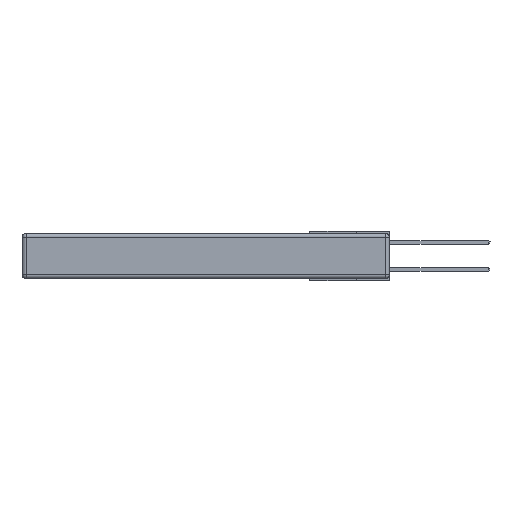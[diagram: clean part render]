
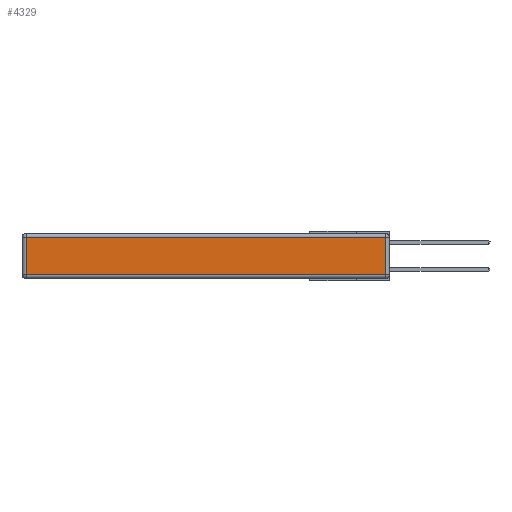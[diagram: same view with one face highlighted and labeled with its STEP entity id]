
A CAD part, left-side view. The second image highlights one B-rep face of the part: STEP entity #4329.
In plain terms, the highlighted planar face has unit normal (-1, 0, 0).
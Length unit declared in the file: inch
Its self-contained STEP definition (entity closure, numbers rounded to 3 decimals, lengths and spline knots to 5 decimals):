
#688 = LINE ( 'NONE', #20197, #33241 ) ;
#1734 = ORIENTED_EDGE ( 'NONE', *, *, #11808, .T. ) ;
#1751 = CARTESIAN_POINT ( 'NONE',  ( 0., 0.03, -0.03 ) ) ;
#2220 = DIRECTION ( 'NONE',  ( -1., 0., 0. ) ) ;
#3815 = DIRECTION ( 'NONE',  ( 0., 0., 1. ) ) ;
#4329 = ADVANCED_FACE ( 'NONE', ( #26496 ), #17851, .T. ) ;
#4511 = CARTESIAN_POINT ( 'NONE',  ( 0., 2.72, -0.313 ) ) ;
#5209 = AXIS2_PLACEMENT_3D ( 'NONE', #18802, #2220, #33996 ) ;
#7578 = ORIENTED_EDGE ( 'NONE', *, *, #8167, .T. ) ;
#8167 = EDGE_CURVE ( 'NONE', #25451, #11094, #35666, .T. ) ;
#9694 = VERTEX_POINT ( 'NONE', #1751 ) ;
#11094 = VERTEX_POINT ( 'NONE', #17493 ) ;
#11808 = EDGE_CURVE ( 'NONE', #9694, #20231, #22403, .T. ) ;
#14972 = EDGE_CURVE ( 'NONE', #20231, #25451, #688, .T. ) ;
#14991 = CARTESIAN_POINT ( 'NONE',  ( 0., 0.03, -0.343 ) ) ;
#17325 = DIRECTION ( 'NONE',  ( 0., -1., 0. ) ) ;
#17493 = CARTESIAN_POINT ( 'NONE',  ( 0., 0.03, -0.313 ) ) ;
#17851 = PLANE ( 'NONE',  #5209 ) ;
#18187 = CARTESIAN_POINT ( 'NONE',  ( 0., 2.75, -0.03 ) ) ;
#18601 = VECTOR ( 'NONE', #3815, 39.37008 ) ;
#18802 = CARTESIAN_POINT ( 'NONE',  ( 0., 0., -0.343 ) ) ;
#19862 = EDGE_CURVE ( 'NONE', #11094, #9694, #22524, .T. ) ;
#20197 = CARTESIAN_POINT ( 'NONE',  ( 0., 2.72, -0.343 ) ) ;
#20231 = VERTEX_POINT ( 'NONE', #34285 ) ;
#22403 = LINE ( 'NONE', #18187, #24816 ) ;
#22524 = LINE ( 'NONE', #14991, #18601 ) ;
#22977 = DIRECTION ( 'NONE',  ( 0., 0., -1. ) ) ;
#23092 = ORIENTED_EDGE ( 'NONE', *, *, #14972, .T. ) ;
#24816 = VECTOR ( 'NONE', #32144, 39.37008 ) ;
#25451 = VERTEX_POINT ( 'NONE', #4511 ) ;
#26059 = ORIENTED_EDGE ( 'NONE', *, *, #19862, .T. ) ;
#26496 = FACE_OUTER_BOUND ( 'NONE', #30833, .T. ) ;
#27394 = VECTOR ( 'NONE', #17325, 39.37008 ) ;
#30833 = EDGE_LOOP ( 'NONE', ( #7578, #26059, #1734, #23092 ) ) ;
#31169 = CARTESIAN_POINT ( 'NONE',  ( 0., 0., -0.313 ) ) ;
#32144 = DIRECTION ( 'NONE',  ( 0., 1., 0. ) ) ;
#33241 = VECTOR ( 'NONE', #22977, 39.37008 ) ;
#33996 = DIRECTION ( 'NONE',  ( 0., 0., 1. ) ) ;
#34285 = CARTESIAN_POINT ( 'NONE',  ( 0., 2.72, -0.03 ) ) ;
#35666 = LINE ( 'NONE', #31169, #27394 ) ;
